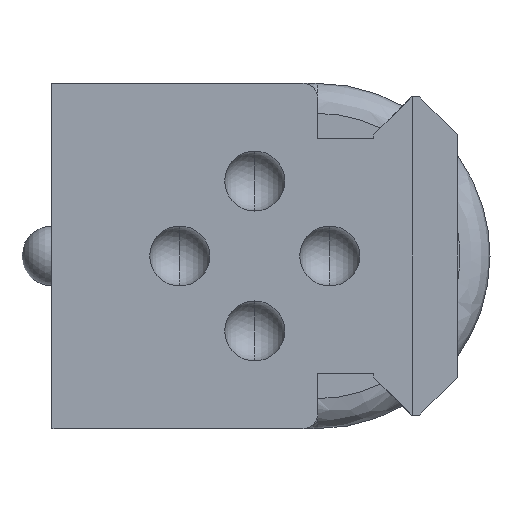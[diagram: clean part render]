
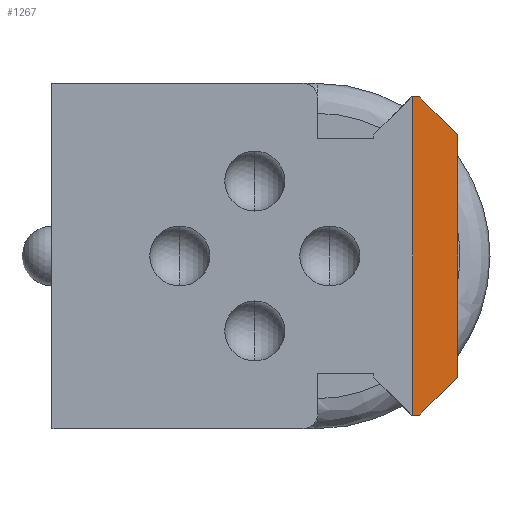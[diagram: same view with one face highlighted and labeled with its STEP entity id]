
A CAD part, front view. The second image highlights one B-rep face of the part: STEP entity #1267.
In plain terms, the highlighted planar face has unit normal (0, -1, 0).
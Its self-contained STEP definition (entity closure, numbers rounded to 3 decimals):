
#28 = EDGE_CURVE ( 'NONE', #2642, #233, #1137, .T. ) ;
#104 = VERTEX_POINT ( 'NONE', #2058 ) ;
#122 = EDGE_CURVE ( 'NONE', #233, #557, #318, .T. ) ;
#156 = DIRECTION ( 'NONE',  ( 0., 0., 1. ) ) ;
#158 = CARTESIAN_POINT ( 'NONE',  ( -98.207, -90.882, -6.057 ) ) ;
#160 = EDGE_CURVE ( 'NONE', #2885, #557, #911, .T. ) ;
#191 = EDGE_LOOP ( 'NONE', ( #1666, #3049, #450, #1096, #2434, #525 ) ) ;
#233 = VERTEX_POINT ( 'NONE', #1773 ) ;
#318 = LINE ( 'NONE', #2049, #3009 ) ;
#432 = CARTESIAN_POINT ( 'NONE',  ( -95.68, -90.882, 15.152 ) ) ;
#450 = ORIENTED_EDGE ( 'NONE', *, *, #160, .T. ) ;
#525 = ORIENTED_EDGE ( 'NONE', *, *, #581, .T. ) ;
#557 = VERTEX_POINT ( 'NONE', #1980 ) ;
#581 = EDGE_CURVE ( 'NONE', #2642, #2338, #1016, .T. ) ;
#665 = CARTESIAN_POINT ( 'NONE',  ( -98.677, -90.882, -6.057 ) ) ;
#825 = CARTESIAN_POINT ( 'NONE',  ( -95.68, -90.882, 12.625 ) ) ;
#826 = VECTOR ( 'NONE', #1844, 1000. ) ;
#909 = CARTESIAN_POINT ( 'NONE',  ( -98.677, -90.882, 15.152 ) ) ;
#911 = LINE ( 'NONE', #1878, #826 ) ;
#995 = VECTOR ( 'NONE', #1801, 1000. ) ;
#1016 = LINE ( 'NONE', #2910, #1497 ) ;
#1019 = DIRECTION ( 'NONE',  ( 1., 0., 0. ) ) ;
#1058 = VECTOR ( 'NONE', #2367, 1000. ) ;
#1096 = ORIENTED_EDGE ( 'NONE', *, *, #122, .F. ) ;
#1137 = LINE ( 'NONE', #2478, #1058 ) ;
#1153 = PLANE ( 'NONE',  #1200 ) ;
#1200 = AXIS2_PLACEMENT_3D ( 'NONE', #909, #1638, #156 ) ;
#1267 = ADVANCED_FACE ( 'NONE', ( #2925 ), #1153, .F. ) ;
#1305 = VECTOR ( 'NONE', #1395, 1000. ) ;
#1321 = EDGE_CURVE ( 'NONE', #104, #2885, #2684, .T. ) ;
#1395 = DIRECTION ( 'NONE',  ( 0., 0., 1. ) ) ;
#1497 = VECTOR ( 'NONE', #1019, 1000. ) ;
#1546 = CARTESIAN_POINT ( 'NONE',  ( -97.102, -90.882, -4.952 ) ) ;
#1638 = DIRECTION ( 'NONE',  ( 0., 1., 0. ) ) ;
#1666 = ORIENTED_EDGE ( 'NONE', *, *, #2870, .T. ) ;
#1773 = CARTESIAN_POINT ( 'NONE',  ( -98.677, -90.882, 15.152 ) ) ;
#1801 = DIRECTION ( 'NONE',  ( 0.707, 0., 0.707 ) ) ;
#1844 = DIRECTION ( 'NONE',  ( -0.707, 0., 0.707 ) ) ;
#1878 = CARTESIAN_POINT ( 'NONE',  ( -97.102, -90.882, 14.047 ) ) ;
#1980 = CARTESIAN_POINT ( 'NONE',  ( -98.207, -90.882, 15.152 ) ) ;
#2031 = DIRECTION ( 'NONE',  ( 1., 0., 0. ) ) ;
#2049 = CARTESIAN_POINT ( 'NONE',  ( -98.677, -90.882, 15.152 ) ) ;
#2058 = CARTESIAN_POINT ( 'NONE',  ( -95.68, -90.882, -3.53 ) ) ;
#2338 = VERTEX_POINT ( 'NONE', #158 ) ;
#2367 = DIRECTION ( 'NONE',  ( 0., 0., 1. ) ) ;
#2398 = LINE ( 'NONE', #1546, #995 ) ;
#2434 = ORIENTED_EDGE ( 'NONE', *, *, #28, .F. ) ;
#2478 = CARTESIAN_POINT ( 'NONE',  ( -98.677, -90.882, 15.152 ) ) ;
#2642 = VERTEX_POINT ( 'NONE', #665 ) ;
#2684 = LINE ( 'NONE', #432, #1305 ) ;
#2870 = EDGE_CURVE ( 'NONE', #2338, #104, #2398, .T. ) ;
#2885 = VERTEX_POINT ( 'NONE', #825 ) ;
#2910 = CARTESIAN_POINT ( 'NONE',  ( -98.677, -90.882, -6.057 ) ) ;
#2925 = FACE_OUTER_BOUND ( 'NONE', #191, .T. ) ;
#3009 = VECTOR ( 'NONE', #2031, 1000. ) ;
#3049 = ORIENTED_EDGE ( 'NONE', *, *, #1321, .T. ) ;
